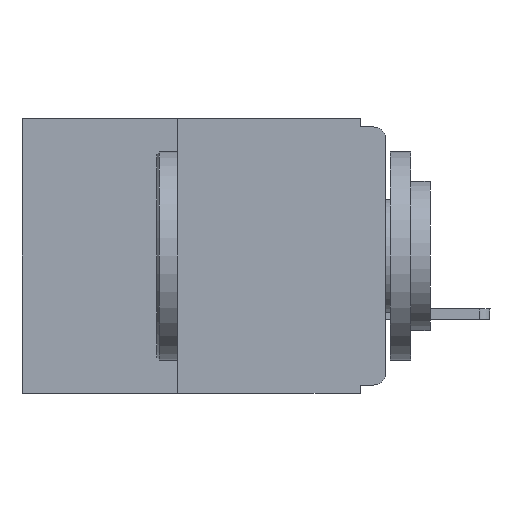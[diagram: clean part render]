
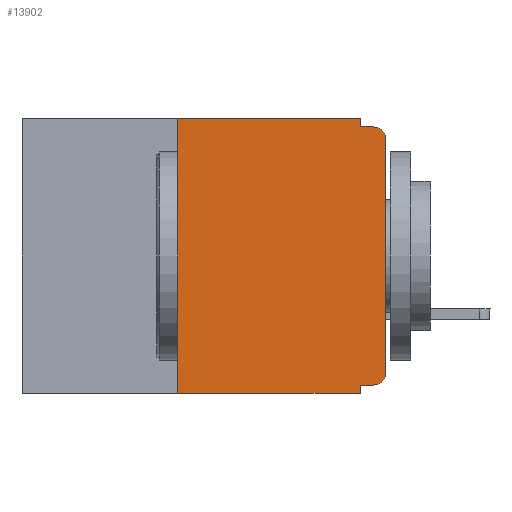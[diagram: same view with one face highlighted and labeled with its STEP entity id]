
A CAD part, left-side view. The second image highlights one B-rep face of the part: STEP entity #13902.
In plain terms, the highlighted planar face has unit normal (-1, 0, 0).
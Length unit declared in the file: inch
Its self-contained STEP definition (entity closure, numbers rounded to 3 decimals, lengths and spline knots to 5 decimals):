
#383 = LINE ( 'NONE', #5258, #8024 ) ;
#388 = PLANE ( 'NONE',  #11876 ) ;
#441 = VERTEX_POINT ( 'NONE', #7241 ) ;
#926 = CARTESIAN_POINT ( 'NONE',  ( 0., 0.031, -0.32 ) ) ;
#999 = LINE ( 'NONE', #3845, #10266 ) ;
#1069 = EDGE_CURVE ( 'NONE', #2210, #11061, #6051, .T. ) ;
#1270 = ORIENTED_EDGE ( 'NONE', *, *, #2911, .T. ) ;
#1413 = VERTEX_POINT ( 'NONE', #6614 ) ;
#1570 = VECTOR ( 'NONE', #5900, 39.37008 ) ;
#1744 = ORIENTED_EDGE ( 'NONE', *, *, #11334, .F. ) ;
#1999 = FACE_OUTER_BOUND ( 'NONE', #11873, .T. ) ;
#2147 = VERTEX_POINT ( 'NONE', #3323 ) ;
#2210 = VERTEX_POINT ( 'NONE', #926 ) ;
#2271 = VERTEX_POINT ( 'NONE', #3695 ) ;
#2596 = VERTEX_POINT ( 'NONE', #10280 ) ;
#2911 = EDGE_CURVE ( 'NONE', #8348, #2271, #6995, .T. ) ;
#3043 = DIRECTION ( 'NONE',  ( 0., -1., 0. ) ) ;
#3096 = DIRECTION ( 'NONE',  ( 0., 0., -1. ) ) ;
#3214 = CARTESIAN_POINT ( 'NONE',  ( 0., 0.031, -0.33 ) ) ;
#3323 = CARTESIAN_POINT ( 'NONE',  ( 0., 0.031, -0.01 ) ) ;
#3475 = DIRECTION ( 'NONE',  ( 0., 0., -1. ) ) ;
#3695 = CARTESIAN_POINT ( 'NONE',  ( 0., 0., -0.305 ) ) ;
#3762 = EDGE_CURVE ( 'NONE', #2596, #10439, #999, .T. ) ;
#3845 = CARTESIAN_POINT ( 'NONE',  ( 0., 0.25, -0.33 ) ) ;
#4365 = DIRECTION ( 'NONE',  ( 0., 0., -1. ) ) ;
#4413 = DIRECTION ( 'NONE',  ( 1., 0., 0. ) ) ;
#4429 = ORIENTED_EDGE ( 'NONE', *, *, #12259, .F. ) ;
#4510 = VECTOR ( 'NONE', #7141, 39.37008 ) ;
#4713 = DIRECTION ( 'NONE',  ( 0., 0., 1. ) ) ;
#4849 = DIRECTION ( 'NONE',  ( -1., 0., 0. ) ) ;
#5223 = DIRECTION ( 'NONE',  ( -1., 0., 0. ) ) ;
#5235 = VECTOR ( 'NONE', #4713, 39.37008 ) ;
#5258 = CARTESIAN_POINT ( 'NONE',  ( 0., 0.437, 0. ) ) ;
#5444 = CARTESIAN_POINT ( 'NONE',  ( 0., 0.437, -0.33 ) ) ;
#5900 = DIRECTION ( 'NONE',  ( 0., -1., 0. ) ) ;
#6051 = LINE ( 'NONE', #3214, #9777 ) ;
#6481 = DIRECTION ( 'NONE',  ( 0., 0., -1. ) ) ;
#6614 = CARTESIAN_POINT ( 'NONE',  ( 0., 0.031, 0. ) ) ;
#6995 = CIRCLE ( 'NONE', #13170, 0.015 ) ;
#7141 = DIRECTION ( 'NONE',  ( 0., 1., 0. ) ) ;
#7241 = CARTESIAN_POINT ( 'NONE',  ( 0., 0.015, -0.01 ) ) ;
#7248 = CARTESIAN_POINT ( 'NONE',  ( 0., 0.031, 0. ) ) ;
#7594 = EDGE_CURVE ( 'NONE', #2596, #11061, #10347, .T. ) ;
#8024 = VECTOR ( 'NONE', #3043, 39.37008 ) ;
#8054 = LINE ( 'NONE', #7248, #13277 ) ;
#8201 = ORIENTED_EDGE ( 'NONE', *, *, #1069, .F. ) ;
#8240 = VERTEX_POINT ( 'NONE', #15406 ) ;
#8348 = VERTEX_POINT ( 'NONE', #17075 ) ;
#8502 = EDGE_CURVE ( 'NONE', #8348, #2210, #11578, .T. ) ;
#8925 = LINE ( 'NONE', #14159, #5235 ) ;
#9003 = DIRECTION ( 'NONE',  ( 0., 0., 1. ) ) ;
#9545 = CIRCLE ( 'NONE', #9573, 0.015 ) ;
#9573 = AXIS2_PLACEMENT_3D ( 'NONE', #14424, #5223, #6481 ) ;
#9574 = EDGE_CURVE ( 'NONE', #2271, #8240, #8925, .T. ) ;
#9609 = CARTESIAN_POINT ( 'NONE',  ( 0., 0.437, 0. ) ) ;
#9777 = VECTOR ( 'NONE', #3096, 39.37008 ) ;
#9789 = ORIENTED_EDGE ( 'NONE', *, *, #10071, .T. ) ;
#9952 = ORIENTED_EDGE ( 'NONE', *, *, #8502, .F. ) ;
#10071 = EDGE_CURVE ( 'NONE', #8240, #441, #9545, .T. ) ;
#10266 = VECTOR ( 'NONE', #9003, 39.37008 ) ;
#10280 = CARTESIAN_POINT ( 'NONE',  ( 0., 0.25, -0.33 ) ) ;
#10347 = LINE ( 'NONE', #5444, #13671 ) ;
#10439 = VERTEX_POINT ( 'NONE', #11995 ) ;
#10485 = ORIENTED_EDGE ( 'NONE', *, *, #9574, .T. ) ;
#11061 = VERTEX_POINT ( 'NONE', #13332 ) ;
#11334 = EDGE_CURVE ( 'NONE', #1413, #2147, #8054, .T. ) ;
#11578 = LINE ( 'NONE', #13719, #4510 ) ;
#11873 = EDGE_LOOP ( 'NONE', ( #10485, #9789, #11964, #1744, #4429, #16467, #14403, #8201, #9952, #1270 ) ) ;
#11876 = AXIS2_PLACEMENT_3D ( 'NONE', #9609, #4413, #4365 ) ;
#11964 = ORIENTED_EDGE ( 'NONE', *, *, #15279, .F. ) ;
#11995 = CARTESIAN_POINT ( 'NONE',  ( 0., 0.25, 0. ) ) ;
#12259 = EDGE_CURVE ( 'NONE', #10439, #1413, #383, .T. ) ;
#12373 = CARTESIAN_POINT ( 'NONE',  ( 0., 0., -0.01 ) ) ;
#13170 = AXIS2_PLACEMENT_3D ( 'NONE', #16805, #4849, #14302 ) ;
#13277 = VECTOR ( 'NONE', #3475, 39.37008 ) ;
#13332 = CARTESIAN_POINT ( 'NONE',  ( 0., 0.031, -0.33 ) ) ;
#13444 = DIRECTION ( 'NONE',  ( 0., -1., 0. ) ) ;
#13671 = VECTOR ( 'NONE', #13444, 39.37008 ) ;
#13719 = CARTESIAN_POINT ( 'NONE',  ( 0., 0., -0.32 ) ) ;
#13902 = ADVANCED_FACE ( 'NONE', ( #1999 ), #388, .F. ) ;
#14159 = CARTESIAN_POINT ( 'NONE',  ( 0., 0., 0. ) ) ;
#14302 = DIRECTION ( 'NONE',  ( 0., 0., -1. ) ) ;
#14403 = ORIENTED_EDGE ( 'NONE', *, *, #7594, .T. ) ;
#14424 = CARTESIAN_POINT ( 'NONE',  ( 0., 0.015, -0.025 ) ) ;
#15279 = EDGE_CURVE ( 'NONE', #2147, #441, #17039, .T. ) ;
#15406 = CARTESIAN_POINT ( 'NONE',  ( 0., 0., -0.025 ) ) ;
#16467 = ORIENTED_EDGE ( 'NONE', *, *, #3762, .F. ) ;
#16805 = CARTESIAN_POINT ( 'NONE',  ( 0., 0.015, -0.305 ) ) ;
#17039 = LINE ( 'NONE', #12373, #1570 ) ;
#17075 = CARTESIAN_POINT ( 'NONE',  ( 0., 0.015, -0.32 ) ) ;
